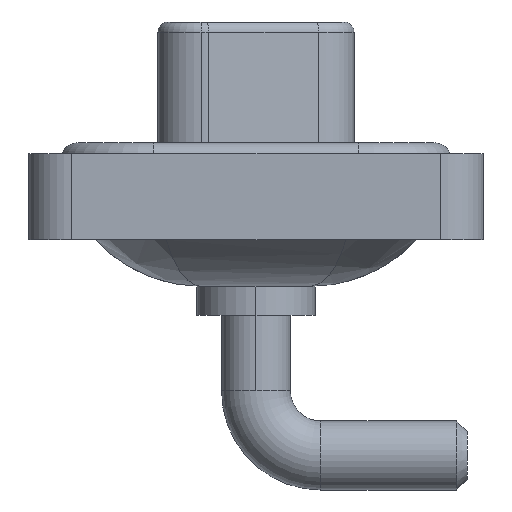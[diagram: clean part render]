
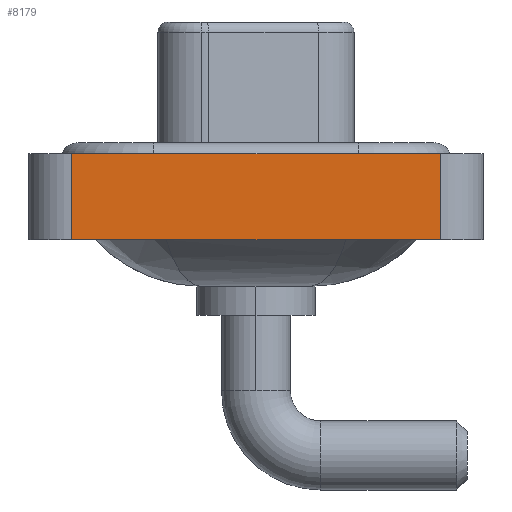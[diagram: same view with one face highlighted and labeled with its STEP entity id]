
A CAD part, left-side view. The second image highlights one B-rep face of the part: STEP entity #8179.
In plain terms, the highlighted planar face has unit normal (-1, 0, 0).
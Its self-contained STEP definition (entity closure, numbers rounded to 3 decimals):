
#349 = VERTEX_POINT ( 'NONE', #2215 ) ;
#757 = FACE_OUTER_BOUND ( 'NONE', #11662, .T. ) ;
#1091 = EDGE_CURVE ( 'NONE', #10069, #349, #6165, .T. ) ;
#1368 = EDGE_CURVE ( 'NONE', #1452, #9535, #15103, .T. ) ;
#1452 = VERTEX_POINT ( 'NONE', #14115 ) ;
#1567 = LINE ( 'NONE', #8533, #13322 ) ;
#1744 = EDGE_CURVE ( 'NONE', #9535, #349, #1567, .T. ) ;
#2122 = CARTESIAN_POINT ( 'NONE',  ( -7.25, -8.55, -3.6 ) ) ;
#2215 = CARTESIAN_POINT ( 'NONE',  ( -7.25, -8.55, 0.4 ) ) ;
#2400 = ORIENTED_EDGE ( 'NONE', *, *, #1091, .F. ) ;
#2669 = ORIENTED_EDGE ( 'NONE', *, *, #3727, .F. ) ;
#2856 = DIRECTION ( 'NONE',  ( 0., 0., 1. ) ) ;
#3307 = DIRECTION ( 'NONE',  ( 0., -1., 0. ) ) ;
#3727 = EDGE_CURVE ( 'NONE', #1452, #10069, #6975, .T. ) ;
#6165 = LINE ( 'NONE', #14502, #12907 ) ;
#6975 = LINE ( 'NONE', #13950, #12354 ) ;
#7276 = VECTOR ( 'NONE', #3307, 1000. ) ;
#7389 = DIRECTION ( 'NONE',  ( 0., -1., 0. ) ) ;
#8007 = PLANE ( 'NONE',  #9655 ) ;
#8053 = DIRECTION ( 'NONE',  ( 0., 0., 1. ) ) ;
#8068 = CARTESIAN_POINT ( 'NONE',  ( -7.25, -8.55, -3.6 ) ) ;
#8179 = ADVANCED_FACE ( 'NONE', ( #757 ), #8007, .T. ) ;
#8533 = CARTESIAN_POINT ( 'NONE',  ( -7.25, -8.55, -3.6 ) ) ;
#9009 = DIRECTION ( 'NONE',  ( 0., 0., 1. ) ) ;
#9149 = ORIENTED_EDGE ( 'NONE', *, *, #1368, .T. ) ;
#9209 = CARTESIAN_POINT ( 'NONE',  ( -7.25, -8.55, -3.6 ) ) ;
#9284 = ORIENTED_EDGE ( 'NONE', *, *, #1744, .T. ) ;
#9535 = VERTEX_POINT ( 'NONE', #8068 ) ;
#9655 = AXIS2_PLACEMENT_3D ( 'NONE', #2122, #14751, #9009 ) ;
#10069 = VERTEX_POINT ( 'NONE', #10739 ) ;
#10739 = CARTESIAN_POINT ( 'NONE',  ( -7.25, 8.55, 0.4 ) ) ;
#11662 = EDGE_LOOP ( 'NONE', ( #9284, #2400, #2669, #9149 ) ) ;
#12354 = VECTOR ( 'NONE', #8053, 1000. ) ;
#12907 = VECTOR ( 'NONE', #7389, 1000. ) ;
#13322 = VECTOR ( 'NONE', #2856, 1000. ) ;
#13950 = CARTESIAN_POINT ( 'NONE',  ( -7.25, 8.55, -3.6 ) ) ;
#14115 = CARTESIAN_POINT ( 'NONE',  ( -7.25, 8.55, -3.6 ) ) ;
#14502 = CARTESIAN_POINT ( 'NONE',  ( -7.25, -8.55, 0.4 ) ) ;
#14751 = DIRECTION ( 'NONE',  ( -1., 0., 0. ) ) ;
#15103 = LINE ( 'NONE', #9209, #7276 ) ;
